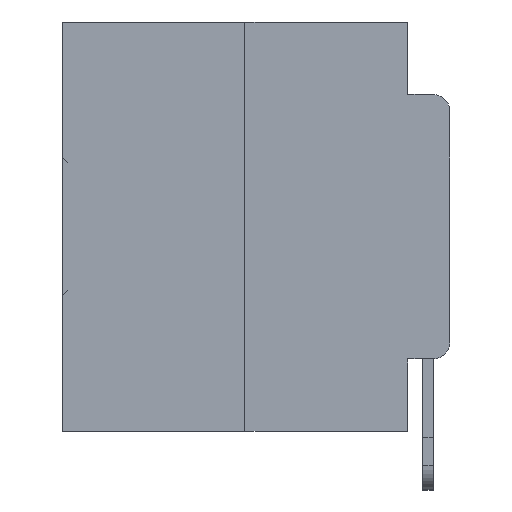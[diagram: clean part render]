
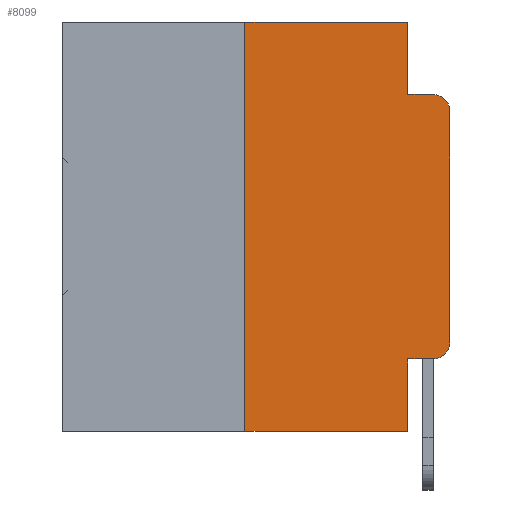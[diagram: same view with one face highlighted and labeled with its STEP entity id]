
A CAD part, left-side view. The second image highlights one B-rep face of the part: STEP entity #8099.
In plain terms, the highlighted planar face has unit normal (-1, 0, 0).
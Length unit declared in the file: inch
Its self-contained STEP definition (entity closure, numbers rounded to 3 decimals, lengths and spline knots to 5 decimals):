
#378 = ORIENTED_EDGE ( 'NONE', *, *, #22749, .F. ) ;
#406 = VERTEX_POINT ( 'NONE', #15749 ) ;
#635 = PLANE ( 'NONE',  #11441 ) ;
#1104 = DIRECTION ( 'NONE',  ( 0., 0., -1. ) ) ;
#1318 = VERTEX_POINT ( 'NONE', #8033 ) ;
#1666 = VERTEX_POINT ( 'NONE', #26481 ) ;
#2410 = DIRECTION ( 'NONE',  ( 0., 0., -1. ) ) ;
#2848 = CARTESIAN_POINT ( 'NONE',  ( 0., 0.051, 0. ) ) ;
#3027 = DIRECTION ( 'NONE',  ( 0., -1., 0. ) ) ;
#3512 = LINE ( 'NONE', #32353, #16587 ) ;
#3748 = EDGE_CURVE ( 'NONE', #16729, #31962, #22140, .T. ) ;
#4199 = VECTOR ( 'NONE', #14598, 39.37008 ) ;
#4355 = CARTESIAN_POINT ( 'NONE',  ( 0., 0., -0.1085 ) ) ;
#6190 = DIRECTION ( 'NONE',  ( 0., 0., -1. ) ) ;
#6402 = EDGE_CURVE ( 'NONE', #23421, #1318, #7362, .T. ) ;
#6441 = ORIENTED_EDGE ( 'NONE', *, *, #18829, .T. ) ;
#7362 = LINE ( 'NONE', #22709, #14294 ) ;
#7480 = DIRECTION ( 'NONE',  ( 0., 0., 1. ) ) ;
#8033 = CARTESIAN_POINT ( 'NONE',  ( 0., 0.02, -0.4115 ) ) ;
#8087 = ORIENTED_EDGE ( 'NONE', *, *, #26842, .F. ) ;
#8099 = ADVANCED_FACE ( 'NONE', ( #18717 ), #635, .F. ) ;
#10841 = LINE ( 'NONE', #26395, #17750 ) ;
#10859 = VECTOR ( 'NONE', #26358, 39.37008 ) ;
#11309 = ORIENTED_EDGE ( 'NONE', *, *, #3748, .F. ) ;
#11441 = AXIS2_PLACEMENT_3D ( 'NONE', #24258, #21800, #6190 ) ;
#11958 = LINE ( 'NONE', #14491, #4199 ) ;
#12159 = ORIENTED_EDGE ( 'NONE', *, *, #27690, .T. ) ;
#12477 = LINE ( 'NONE', #2848, #10859 ) ;
#12731 = CARTESIAN_POINT ( 'NONE',  ( 0., 0.051, 0. ) ) ;
#13151 = VECTOR ( 'NONE', #22715, 39.37008 ) ;
#13402 = EDGE_CURVE ( 'NONE', #1318, #1666, #28028, .T. ) ;
#13820 = CIRCLE ( 'NONE', #16460, 0.02 ) ;
#13975 = VECTOR ( 'NONE', #7480, 39.37008 ) ;
#14294 = VECTOR ( 'NONE', #25267, 39.37008 ) ;
#14491 = CARTESIAN_POINT ( 'NONE',  ( 0., 0.051, -0.0885 ) ) ;
#14598 = DIRECTION ( 'NONE',  ( 0., -1., 0. ) ) ;
#15020 = EDGE_CURVE ( 'NONE', #26584, #406, #10841, .T. ) ;
#15316 = VERTEX_POINT ( 'NONE', #4355 ) ;
#15517 = DIRECTION ( 'NONE',  ( -1., 0., 0. ) ) ;
#15749 = CARTESIAN_POINT ( 'NONE',  ( 0., 0.051, -0.5 ) ) ;
#16208 = ORIENTED_EDGE ( 'NONE', *, *, #15020, .T. ) ;
#16460 = AXIS2_PLACEMENT_3D ( 'NONE', #30960, #15517, #33487 ) ;
#16587 = VECTOR ( 'NONE', #1104, 39.37008 ) ;
#16729 = VERTEX_POINT ( 'NONE', #22989 ) ;
#17750 = VECTOR ( 'NONE', #3027, 39.37008 ) ;
#18190 = DIRECTION ( 'NONE',  ( -1., 0., 0. ) ) ;
#18717 = FACE_OUTER_BOUND ( 'NONE', #24605, .T. ) ;
#18829 = EDGE_CURVE ( 'NONE', #15316, #20885, #13820, .T. ) ;
#19520 = ORIENTED_EDGE ( 'NONE', *, *, #24446, .F. ) ;
#20109 = CARTESIAN_POINT ( 'NONE',  ( 0., 0.25, 0. ) ) ;
#20885 = VERTEX_POINT ( 'NONE', #27701 ) ;
#20887 = LINE ( 'NONE', #23052, #13975 ) ;
#21331 = VECTOR ( 'NONE', #33165, 39.37008 ) ;
#21680 = VERTEX_POINT ( 'NONE', #33375 ) ;
#21800 = DIRECTION ( 'NONE',  ( 1., 0., 0. ) ) ;
#22140 = LINE ( 'NONE', #28113, #21331 ) ;
#22709 = CARTESIAN_POINT ( 'NONE',  ( 0., 0.051, -0.4115 ) ) ;
#22715 = DIRECTION ( 'NONE',  ( 0., 0., 1. ) ) ;
#22749 = EDGE_CURVE ( 'NONE', #31962, #21680, #12477, .T. ) ;
#22989 = CARTESIAN_POINT ( 'NONE',  ( 0., 0.25, 0. ) ) ;
#23052 = CARTESIAN_POINT ( 'NONE',  ( 0., 0., 0. ) ) ;
#23421 = VERTEX_POINT ( 'NONE', #26382 ) ;
#24258 = CARTESIAN_POINT ( 'NONE',  ( 0., 0.473, 0. ) ) ;
#24446 = EDGE_CURVE ( 'NONE', #26584, #16729, #33639, .T. ) ;
#24605 = EDGE_LOOP ( 'NONE', ( #12159, #6441, #8087, #378, #11309, #19520, #16208, #27596, #28985, #30557 ) ) ;
#25267 = DIRECTION ( 'NONE',  ( 0., -1., 0. ) ) ;
#26358 = DIRECTION ( 'NONE',  ( 0., 0., -1. ) ) ;
#26382 = CARTESIAN_POINT ( 'NONE',  ( 0., 0.051, -0.4115 ) ) ;
#26395 = CARTESIAN_POINT ( 'NONE',  ( 0., 0.473, -0.5 ) ) ;
#26481 = CARTESIAN_POINT ( 'NONE',  ( 0., 0., -0.3915 ) ) ;
#26493 = CARTESIAN_POINT ( 'NONE',  ( 0., 0.25, -0.5 ) ) ;
#26584 = VERTEX_POINT ( 'NONE', #26493 ) ;
#26842 = EDGE_CURVE ( 'NONE', #21680, #20885, #11958, .T. ) ;
#27596 = ORIENTED_EDGE ( 'NONE', *, *, #32995, .F. ) ;
#27690 = EDGE_CURVE ( 'NONE', #1666, #15316, #20887, .T. ) ;
#27701 = CARTESIAN_POINT ( 'NONE',  ( 0., 0.02, -0.0885 ) ) ;
#28028 = CIRCLE ( 'NONE', #33283, 0.02 ) ;
#28113 = CARTESIAN_POINT ( 'NONE',  ( 0., 0.473, 0. ) ) ;
#28985 = ORIENTED_EDGE ( 'NONE', *, *, #6402, .T. ) ;
#30557 = ORIENTED_EDGE ( 'NONE', *, *, #13402, .T. ) ;
#30960 = CARTESIAN_POINT ( 'NONE',  ( 0., 0.02, -0.1085 ) ) ;
#31962 = VERTEX_POINT ( 'NONE', #12731 ) ;
#32353 = CARTESIAN_POINT ( 'NONE',  ( 0., 0.051, 0. ) ) ;
#32995 = EDGE_CURVE ( 'NONE', #23421, #406, #3512, .T. ) ;
#33165 = DIRECTION ( 'NONE',  ( 0., -1., 0. ) ) ;
#33283 = AXIS2_PLACEMENT_3D ( 'NONE', #33501, #18190, #2410 ) ;
#33375 = CARTESIAN_POINT ( 'NONE',  ( 0., 0.051, -0.0885 ) ) ;
#33487 = DIRECTION ( 'NONE',  ( 0., 0., -1. ) ) ;
#33501 = CARTESIAN_POINT ( 'NONE',  ( 0., 0.02, -0.3915 ) ) ;
#33639 = LINE ( 'NONE', #20109, #13151 ) ;
